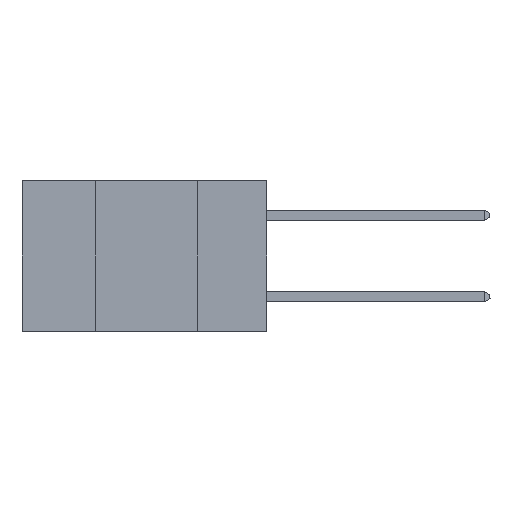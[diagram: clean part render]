
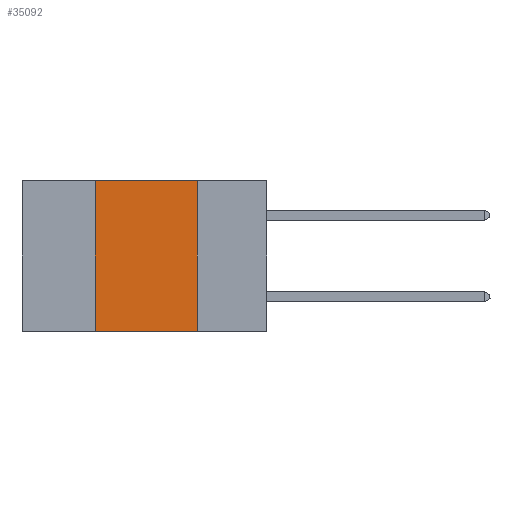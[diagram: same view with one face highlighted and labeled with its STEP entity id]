
A CAD part, left-side view. The second image highlights one B-rep face of the part: STEP entity #35092.
In plain terms, the highlighted planar face has unit normal (-1, 0, 0).
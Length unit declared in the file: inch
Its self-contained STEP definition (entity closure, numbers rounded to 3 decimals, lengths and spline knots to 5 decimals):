
#140 = VECTOR ( 'NONE', #33531, 39.37008 ) ;
#2650 = CARTESIAN_POINT ( 'NONE',  ( 0., 0.42, 0. ) ) ;
#3911 = VERTEX_POINT ( 'NONE', #45151 ) ;
#3936 = DIRECTION ( 'NONE',  ( 0., 0., 1. ) ) ;
#4424 = DIRECTION ( 'NONE',  ( 0., 0., -1. ) ) ;
#5645 = EDGE_CURVE ( 'NONE', #3911, #9743, #22559, .T. ) ;
#6970 = ORIENTED_EDGE ( 'NONE', *, *, #33538, .T. ) ;
#8693 = EDGE_CURVE ( 'NONE', #9743, #46360, #12507, .T. ) ;
#8736 = LINE ( 'NONE', #14153, #45577 ) ;
#9253 = ORIENTED_EDGE ( 'NONE', *, *, #8693, .F. ) ;
#9743 = VERTEX_POINT ( 'NONE', #2650 ) ;
#12507 = LINE ( 'NONE', #20900, #13689 ) ;
#12758 = VERTEX_POINT ( 'NONE', #31730 ) ;
#13689 = VECTOR ( 'NONE', #45289, 39.37008 ) ;
#14153 = CARTESIAN_POINT ( 'NONE',  ( 0., 0.17, 0. ) ) ;
#14817 = EDGE_CURVE ( 'NONE', #46360, #12758, #8736, .T. ) ;
#18311 = AXIS2_PLACEMENT_3D ( 'NONE', #43967, #26785, #4424 ) ;
#20900 = CARTESIAN_POINT ( 'NONE',  ( 0., 0.6, 0. ) ) ;
#22559 = LINE ( 'NONE', #26354, #22873 ) ;
#22873 = VECTOR ( 'NONE', #3936, 39.37008 ) ;
#23128 = PLANE ( 'NONE',  #18311 ) ;
#24327 = EDGE_LOOP ( 'NONE', ( #41954, #9253, #27108, #6970 ) ) ;
#26354 = CARTESIAN_POINT ( 'NONE',  ( 0., 0.42, 0. ) ) ;
#26572 = CARTESIAN_POINT ( 'NONE',  ( 0., 0.6, -0.37 ) ) ;
#26785 = DIRECTION ( 'NONE',  ( 1., 0., 0. ) ) ;
#27108 = ORIENTED_EDGE ( 'NONE', *, *, #5645, .F. ) ;
#28750 = LINE ( 'NONE', #26572, #140 ) ;
#28910 = DIRECTION ( 'NONE',  ( 0., 0., -1. ) ) ;
#31730 = CARTESIAN_POINT ( 'NONE',  ( 0., 0.17, -0.37 ) ) ;
#33531 = DIRECTION ( 'NONE',  ( 0., -1., 0. ) ) ;
#33538 = EDGE_CURVE ( 'NONE', #3911, #12758, #28750, .T. ) ;
#35092 = ADVANCED_FACE ( 'NONE', ( #42944 ), #23128, .F. ) ;
#39261 = CARTESIAN_POINT ( 'NONE',  ( 0., 0.17, 0. ) ) ;
#41954 = ORIENTED_EDGE ( 'NONE', *, *, #14817, .F. ) ;
#42944 = FACE_OUTER_BOUND ( 'NONE', #24327, .T. ) ;
#43967 = CARTESIAN_POINT ( 'NONE',  ( 0., 0.6, 0. ) ) ;
#45151 = CARTESIAN_POINT ( 'NONE',  ( 0., 0.42, -0.37 ) ) ;
#45289 = DIRECTION ( 'NONE',  ( 0., -1., 0. ) ) ;
#45577 = VECTOR ( 'NONE', #28910, 39.37008 ) ;
#46360 = VERTEX_POINT ( 'NONE', #39261 ) ;
